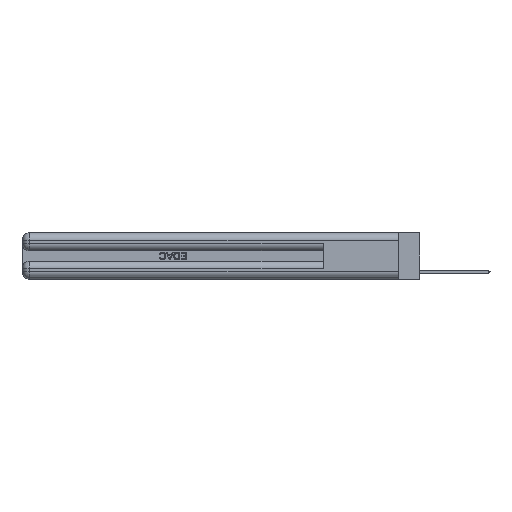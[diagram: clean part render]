
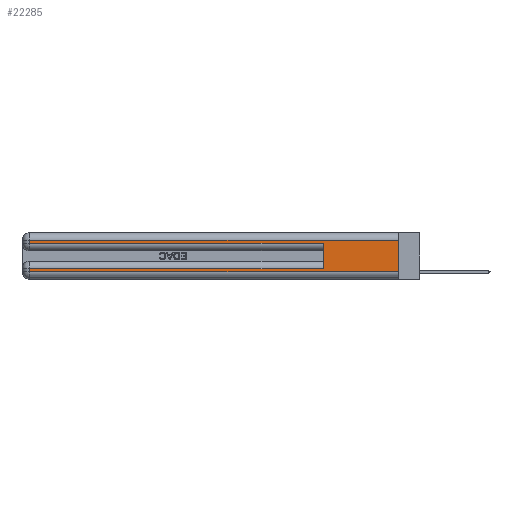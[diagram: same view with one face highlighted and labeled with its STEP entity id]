
A CAD part, left-side view. The second image highlights one B-rep face of the part: STEP entity #22285.
In plain terms, the highlighted planar face has unit normal (-1, 0, 0).
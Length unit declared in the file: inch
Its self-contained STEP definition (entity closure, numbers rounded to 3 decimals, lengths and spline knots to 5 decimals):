
#443 = CARTESIAN_POINT ( 'NONE',  ( 0., 0., 0.31 ) ) ;
#859 = VECTOR ( 'NONE', #3617, 39.37008 ) ;
#1631 = VERTEX_POINT ( 'NONE', #11838 ) ;
#2233 = ORIENTED_EDGE ( 'NONE', *, *, #18493, .T. ) ;
#3116 = VECTOR ( 'NONE', #27491, 39.37008 ) ;
#3617 = DIRECTION ( 'NONE',  ( 0., 1., 0. ) ) ;
#3624 = VERTEX_POINT ( 'NONE', #443 ) ;
#3665 = LINE ( 'NONE', #8786, #7306 ) ;
#3666 = ORIENTED_EDGE ( 'NONE', *, *, #24987, .F. ) ;
#4018 = VERTEX_POINT ( 'NONE', #24699 ) ;
#4605 = ORIENTED_EDGE ( 'NONE', *, *, #16678, .T. ) ;
#4969 = LINE ( 'NONE', #17666, #3116 ) ;
#5258 = LINE ( 'NONE', #28557, #859 ) ;
#6132 = LINE ( 'NONE', #18201, #29256 ) ;
#6434 = VECTOR ( 'NONE', #9878, 39.37008 ) ;
#6643 = ORIENTED_EDGE ( 'NONE', *, *, #30293, .F. ) ;
#6673 = EDGE_CURVE ( 'NONE', #25883, #14849, #5258, .T. ) ;
#6820 = CARTESIAN_POINT ( 'NONE',  ( 0., 2.94, 0.06 ) ) ;
#6877 = CARTESIAN_POINT ( 'NONE',  ( 0., 2.94, 0.37 ) ) ;
#6892 = VERTEX_POINT ( 'NONE', #6820 ) ;
#7306 = VECTOR ( 'NONE', #18623, 39.37008 ) ;
#7777 = DIRECTION ( 'NONE',  ( 0., 0., 1. ) ) ;
#8786 = CARTESIAN_POINT ( 'NONE',  ( 0., 0., 0.31 ) ) ;
#9024 = DIRECTION ( 'NONE',  ( 0., -1., 0. ) ) ;
#9878 = DIRECTION ( 'NONE',  ( 0., 0., -1. ) ) ;
#9880 = ORIENTED_EDGE ( 'NONE', *, *, #19303, .T. ) ;
#10185 = CARTESIAN_POINT ( 'NONE',  ( 0., 0.6, 0.145 ) ) ;
#10205 = CARTESIAN_POINT ( 'NONE',  ( 0., 0., 0.37 ) ) ;
#10511 = FACE_OUTER_BOUND ( 'NONE', #17890, .T. ) ;
#11459 = LINE ( 'NONE', #18553, #16827 ) ;
#11838 = CARTESIAN_POINT ( 'NONE',  ( 0., 2.94, 0.285 ) ) ;
#12014 = DIRECTION ( 'NONE',  ( 0., 0., -1. ) ) ;
#13376 = CARTESIAN_POINT ( 'NONE',  ( 0., 0.6, 0.085 ) ) ;
#13674 = DIRECTION ( 'NONE',  ( 0., -1., 0. ) ) ;
#13792 = CARTESIAN_POINT ( 'NONE',  ( 0., 0.6, 0.285 ) ) ;
#14849 = VERTEX_POINT ( 'NONE', #23650 ) ;
#15362 = DIRECTION ( 'NONE',  ( 1., 0., 0. ) ) ;
#16678 = EDGE_CURVE ( 'NONE', #3624, #4018, #3665, .T. ) ;
#16827 = VECTOR ( 'NONE', #9024, 39.37008 ) ;
#17666 = CARTESIAN_POINT ( 'NONE',  ( 0., 0., 0.37 ) ) ;
#17890 = EDGE_LOOP ( 'NONE', ( #3666, #4605, #2233, #31704, #6643, #25170, #9880, #19049 ) ) ;
#17901 = AXIS2_PLACEMENT_3D ( 'NONE', #10205, #15362, #25173 ) ;
#18201 = CARTESIAN_POINT ( 'NONE',  ( 0., 0., 0.06 ) ) ;
#18493 = EDGE_CURVE ( 'NONE', #4018, #1631, #29539, .T. ) ;
#18553 = CARTESIAN_POINT ( 'NONE',  ( 0., 0., 0.285 ) ) ;
#18623 = DIRECTION ( 'NONE',  ( 0., 1., 0. ) ) ;
#19049 = ORIENTED_EDGE ( 'NONE', *, *, #22872, .T. ) ;
#19195 = VERTEX_POINT ( 'NONE', #13792 ) ;
#19303 = EDGE_CURVE ( 'NONE', #14849, #6892, #19424, .T. ) ;
#19424 = LINE ( 'NONE', #6877, #29694 ) ;
#19548 = EDGE_CURVE ( 'NONE', #1631, #19195, #11459, .T. ) ;
#21245 = VECTOR ( 'NONE', #7777, 39.37008 ) ;
#22285 = ADVANCED_FACE ( 'NONE', ( #10511 ), #29713, .F. ) ;
#22428 = LINE ( 'NONE', #10185, #21245 ) ;
#22872 = EDGE_CURVE ( 'NONE', #6892, #23899, #6132, .T. ) ;
#23650 = CARTESIAN_POINT ( 'NONE',  ( 0., 2.94, 0.085 ) ) ;
#23899 = VERTEX_POINT ( 'NONE', #26319 ) ;
#24699 = CARTESIAN_POINT ( 'NONE',  ( 0., 2.94, 0.31 ) ) ;
#24987 = EDGE_CURVE ( 'NONE', #3624, #23899, #4969, .T. ) ;
#25170 = ORIENTED_EDGE ( 'NONE', *, *, #6673, .T. ) ;
#25173 = DIRECTION ( 'NONE',  ( 0., 0., -1. ) ) ;
#25883 = VERTEX_POINT ( 'NONE', #13376 ) ;
#26319 = CARTESIAN_POINT ( 'NONE',  ( 0., 0., 0.06 ) ) ;
#27280 = CARTESIAN_POINT ( 'NONE',  ( 0., 2.94, 0.37 ) ) ;
#27491 = DIRECTION ( 'NONE',  ( 0., 0., -1. ) ) ;
#28557 = CARTESIAN_POINT ( 'NONE',  ( 0., 0., 0.085 ) ) ;
#29256 = VECTOR ( 'NONE', #13674, 39.37008 ) ;
#29539 = LINE ( 'NONE', #27280, #6434 ) ;
#29694 = VECTOR ( 'NONE', #12014, 39.37008 ) ;
#29713 = PLANE ( 'NONE',  #17901 ) ;
#30293 = EDGE_CURVE ( 'NONE', #25883, #19195, #22428, .T. ) ;
#31704 = ORIENTED_EDGE ( 'NONE', *, *, #19548, .T. ) ;
